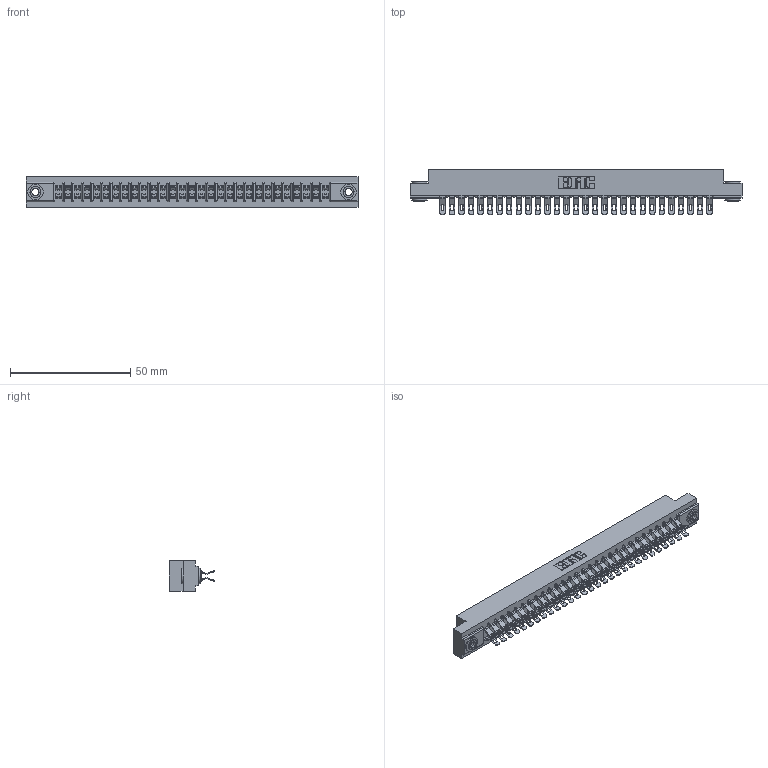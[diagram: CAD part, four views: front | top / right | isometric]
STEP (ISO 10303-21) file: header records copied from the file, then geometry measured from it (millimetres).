
FILE_DESCRIPTION (( 'STEP AP203' ), '1' );
FILE_NAME ('357-058-555-203.STEP', '2018-08-12T14:18:35', ( '' ), ( '' ), 'SwSTEP 2.0', 'SolidWorks 2016', '' );
FILE_SCHEMA (( 'CONFIG_CONTROL_DESIGN' ));
Length unit declared in the file: inch
Products named in the file (4): 345-250-002_345-250-002-102; 357-058-555-203; 307 Part_.156 Dia Mounting Holes; 307-290-001_555
Assembly tree (61 placements, depth 2):
  357-058-555-203
    307 Part_.156 Dia Mounting Holes
    307-290-001_555  x58
    345-250-002_345-250-002-102  x2
Bounding box: 137.92 x 18.75 x 12.7 mm (x, y, z)
Volume: 14748.4 mm3; surface area: 18992.7 mm2
Topology: 61 solids, 61 shells, 3738 faces, 10933 edges, 7126 vertices
Faces by surface type: plane 2066, cylinder 1604, sphere 60, cone 8
Entity records: 28994 total; most frequent: CARTESIAN_POINT 4734, ORIENTED_EDGE 4684, DIRECTION 4664, EDGE_CURVE 2342, LINE 1772, VECTOR 1772, VERTEX_POINT 1516, AXIS2_PLACEMENT_3D 1446
